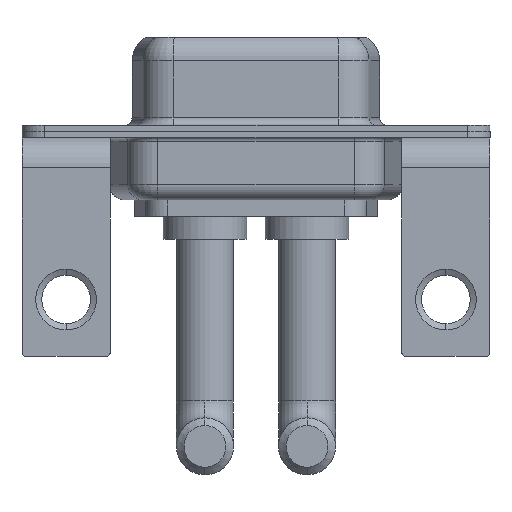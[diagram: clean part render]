
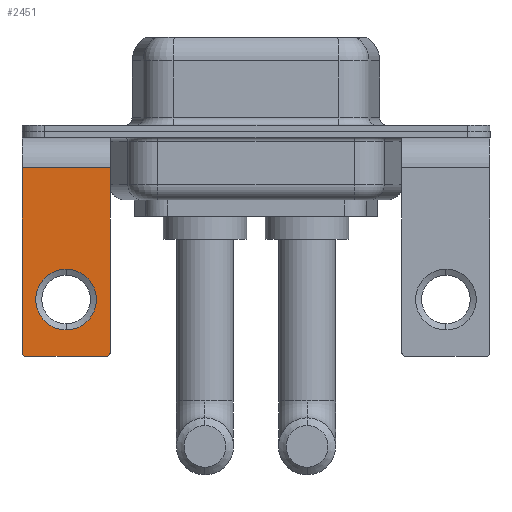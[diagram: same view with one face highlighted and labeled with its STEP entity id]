
A CAD part, front view. The second image highlights one B-rep face of the part: STEP entity #2451.
In plain terms, the highlighted planar face has unit normal (0, -1, 0).
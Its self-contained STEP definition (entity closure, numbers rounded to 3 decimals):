
#415 = CARTESIAN_POINT ( 'NONE',  ( 2.65, -6.25, -14.55 ) ) ;
#526 = AXIS2_PLACEMENT_3D ( 'NONE', #7157, #7958, #9207 ) ;
#746 = ORIENTED_EDGE ( 'NONE', *, *, #1834, .T. ) ;
#837 = VERTEX_POINT ( 'NONE', #12756 ) ;
#910 = VERTEX_POINT ( 'NONE', #11106 ) ;
#975 = CARTESIAN_POINT ( 'NONE',  ( -2.65, -6.25, -14.55 ) ) ;
#1214 = CARTESIAN_POINT ( 'NONE',  ( 2.65, -6.25, -14.8 ) ) ;
#1485 = EDGE_CURVE ( 'NONE', #12293, #8123, #8247, .T. ) ;
#1834 = EDGE_CURVE ( 'NONE', #7876, #910, #12011, .T. ) ;
#1850 = CIRCLE ( 'NONE', #2895, 0.25 ) ;
#2012 = LINE ( 'NONE', #11960, #4353 ) ;
#2451 = ADVANCED_FACE ( 'NONE', ( #9078, #6249 ), #7164, .F. ) ;
#2632 = CARTESIAN_POINT ( 'NONE',  ( -2.65, -6.25, -14.8 ) ) ;
#2895 = AXIS2_PLACEMENT_3D ( 'NONE', #415, #9313, #4256 ) ;
#2919 = CARTESIAN_POINT ( 'NONE',  ( 2.9, -6.25, -14.8 ) ) ;
#2954 = ORIENTED_EDGE ( 'NONE', *, *, #7814, .T. ) ;
#2975 = CARTESIAN_POINT ( 'NONE',  ( 0., -6.25, -11.07 ) ) ;
#3004 = VECTOR ( 'NONE', #11698, 1000. ) ;
#3063 = EDGE_LOOP ( 'NONE', ( #7674, #8625, #3900, #3201, #9244, #2954 ) ) ;
#3201 = ORIENTED_EDGE ( 'NONE', *, *, #7025, .T. ) ;
#3314 = EDGE_CURVE ( 'NONE', #4550, #6690, #5748, .T. ) ;
#3562 = AXIS2_PLACEMENT_3D ( 'NONE', #975, #6205, #12211 ) ;
#3700 = EDGE_CURVE ( 'NONE', #910, #7876, #4279, .T. ) ;
#3900 = ORIENTED_EDGE ( 'NONE', *, *, #3314, .F. ) ;
#3996 = CARTESIAN_POINT ( 'NONE',  ( -2.9, -6.25, -2.4 ) ) ;
#4256 = DIRECTION ( 'NONE',  ( 0., 0., 1. ) ) ;
#4279 = CIRCLE ( 'NONE', #526, 2. ) ;
#4353 = VECTOR ( 'NONE', #5945, 1000. ) ;
#4550 = VERTEX_POINT ( 'NONE', #1214 ) ;
#4613 = CIRCLE ( 'NONE', #3562, 0.25 ) ;
#5748 = LINE ( 'NONE', #2919, #3004 ) ;
#5932 = ORIENTED_EDGE ( 'NONE', *, *, #3700, .T. ) ;
#5945 = DIRECTION ( 'NONE',  ( 0., 0., -1. ) ) ;
#6145 = CARTESIAN_POINT ( 'NONE',  ( -2.9, -6.25, -2.4 ) ) ;
#6205 = DIRECTION ( 'NONE',  ( 0., -1., 0. ) ) ;
#6249 = FACE_OUTER_BOUND ( 'NONE', #3063, .T. ) ;
#6396 = CARTESIAN_POINT ( 'NONE',  ( 2.9, -6.25, -14.55 ) ) ;
#6471 = VECTOR ( 'NONE', #6637, 1000. ) ;
#6566 = AXIS2_PLACEMENT_3D ( 'NONE', #2975, #10979, #6869 ) ;
#6637 = DIRECTION ( 'NONE',  ( -1., 0., 0. ) ) ;
#6690 = VERTEX_POINT ( 'NONE', #2632 ) ;
#6869 = DIRECTION ( 'NONE',  ( 0., 0., 1. ) ) ;
#7025 = EDGE_CURVE ( 'NONE', #4550, #12002, #1850, .T. ) ;
#7157 = CARTESIAN_POINT ( 'NONE',  ( 0., -6.25, -11.07 ) ) ;
#7164 = PLANE ( 'NONE',  #8060 ) ;
#7495 = CARTESIAN_POINT ( 'NONE',  ( 0., -6.25, -13.07 ) ) ;
#7674 = ORIENTED_EDGE ( 'NONE', *, *, #1485, .T. ) ;
#7814 = EDGE_CURVE ( 'NONE', #837, #12293, #9457, .T. ) ;
#7876 = VERTEX_POINT ( 'NONE', #7495 ) ;
#7958 = DIRECTION ( 'NONE',  ( 0., 1., 0. ) ) ;
#8025 = DIRECTION ( 'NONE',  ( 0., 0., 1. ) ) ;
#8060 = AXIS2_PLACEMENT_3D ( 'NONE', #10226, #10089, #8025 ) ;
#8123 = VERTEX_POINT ( 'NONE', #12115 ) ;
#8247 = LINE ( 'NONE', #6145, #11370 ) ;
#8546 = CARTESIAN_POINT ( 'NONE',  ( 2.9, -6.25, -2.4 ) ) ;
#8552 = EDGE_LOOP ( 'NONE', ( #746, #5932 ) ) ;
#8625 = ORIENTED_EDGE ( 'NONE', *, *, #9047, .T. ) ;
#9047 = EDGE_CURVE ( 'NONE', #8123, #6690, #4613, .T. ) ;
#9078 = FACE_BOUND ( 'NONE', #8552, .T. ) ;
#9207 = DIRECTION ( 'NONE',  ( 0., 0., 1. ) ) ;
#9244 = ORIENTED_EDGE ( 'NONE', *, *, #11445, .F. ) ;
#9313 = DIRECTION ( 'NONE',  ( 0., -1., 0. ) ) ;
#9457 = LINE ( 'NONE', #8546, #6471 ) ;
#10089 = DIRECTION ( 'NONE',  ( 0., 1., 0. ) ) ;
#10125 = DIRECTION ( 'NONE',  ( 0., 0., -1. ) ) ;
#10226 = CARTESIAN_POINT ( 'NONE',  ( 2.9, -6.25, -2.4 ) ) ;
#10979 = DIRECTION ( 'NONE',  ( 0., 1., 0. ) ) ;
#11106 = CARTESIAN_POINT ( 'NONE',  ( 0., -6.25, -9.07 ) ) ;
#11370 = VECTOR ( 'NONE', #10125, 1000. ) ;
#11445 = EDGE_CURVE ( 'NONE', #837, #12002, #2012, .T. ) ;
#11698 = DIRECTION ( 'NONE',  ( -1., 0., 0. ) ) ;
#11960 = CARTESIAN_POINT ( 'NONE',  ( 2.9, -6.25, -2.4 ) ) ;
#12002 = VERTEX_POINT ( 'NONE', #6396 ) ;
#12011 = CIRCLE ( 'NONE', #6566, 2. ) ;
#12115 = CARTESIAN_POINT ( 'NONE',  ( -2.9, -6.25, -14.55 ) ) ;
#12211 = DIRECTION ( 'NONE',  ( 0., 0., 1. ) ) ;
#12293 = VERTEX_POINT ( 'NONE', #3996 ) ;
#12756 = CARTESIAN_POINT ( 'NONE',  ( 2.9, -6.25, -2.4 ) ) ;
